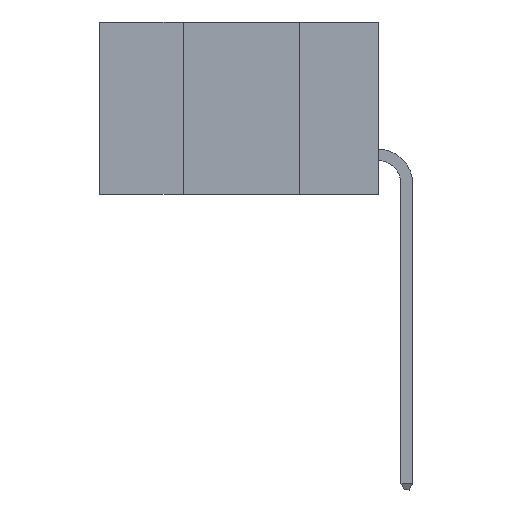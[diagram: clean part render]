
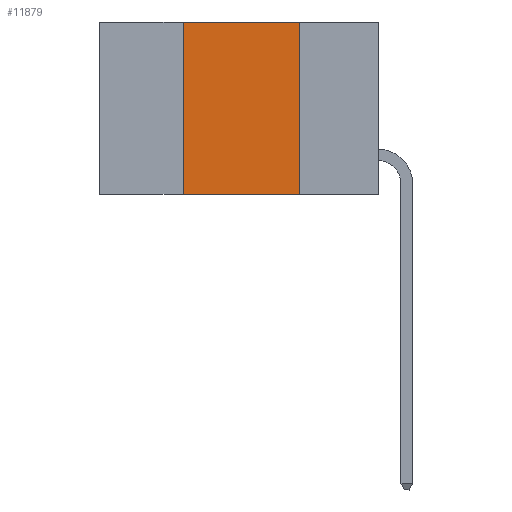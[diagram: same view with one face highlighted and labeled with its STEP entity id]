
A CAD part, left-side view. The second image highlights one B-rep face of the part: STEP entity #11879.
In plain terms, the highlighted planar face has unit normal (-1, 0, 0).
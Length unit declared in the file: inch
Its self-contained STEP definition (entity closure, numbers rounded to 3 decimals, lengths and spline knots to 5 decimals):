
#529 = VERTEX_POINT ( 'NONE', #8936 ) ;
#1614 = DIRECTION ( 'NONE',  ( 1., 0., 0. ) ) ;
#1861 = DIRECTION ( 'NONE',  ( 0., -1., 0. ) ) ;
#1899 = DIRECTION ( 'NONE',  ( 0., 0., -1. ) ) ;
#2452 = VECTOR ( 'NONE', #13883, 39.37008 ) ;
#2727 = EDGE_CURVE ( 'NONE', #3364, #13412, #4231, .T. ) ;
#3364 = VERTEX_POINT ( 'NONE', #25128 ) ;
#3997 = DIRECTION ( 'NONE',  ( 0., -1., 0. ) ) ;
#4231 = LINE ( 'NONE', #13384, #15746 ) ;
#4627 = CARTESIAN_POINT ( 'NONE',  ( 0., 0.17, 0. ) ) ;
#4944 = AXIS2_PLACEMENT_3D ( 'NONE', #15744, #1614, #1899 ) ;
#6671 = VECTOR ( 'NONE', #9051, 39.37008 ) ;
#7128 = VERTEX_POINT ( 'NONE', #12158 ) ;
#7624 = CARTESIAN_POINT ( 'NONE',  ( 0., 0.17, 0. ) ) ;
#8653 = FACE_OUTER_BOUND ( 'NONE', #9447, .T. ) ;
#8936 = CARTESIAN_POINT ( 'NONE',  ( 0., 0.42, -0.37 ) ) ;
#9051 = DIRECTION ( 'NONE',  ( 0., 0., 1. ) ) ;
#9306 = EDGE_CURVE ( 'NONE', #529, #3364, #20756, .T. ) ;
#9447 = EDGE_LOOP ( 'NONE', ( #17401, #18548, #25231, #12040 ) ) ;
#11284 = CARTESIAN_POINT ( 'NONE',  ( 0., 0.42, 0. ) ) ;
#11879 = ADVANCED_FACE ( 'NONE', ( #8653 ), #24726, .F. ) ;
#12040 = ORIENTED_EDGE ( 'NONE', *, *, #18620, .T. ) ;
#12158 = CARTESIAN_POINT ( 'NONE',  ( 0., 0.17, -0.37 ) ) ;
#13384 = CARTESIAN_POINT ( 'NONE',  ( 0., 0.6, 0. ) ) ;
#13412 = VERTEX_POINT ( 'NONE', #7624 ) ;
#13883 = DIRECTION ( 'NONE',  ( 0., 0., -1. ) ) ;
#15744 = CARTESIAN_POINT ( 'NONE',  ( 0., 0.6, 0. ) ) ;
#15746 = VECTOR ( 'NONE', #1861, 39.37008 ) ;
#17379 = CARTESIAN_POINT ( 'NONE',  ( 0., 0.6, -0.37 ) ) ;
#17401 = ORIENTED_EDGE ( 'NONE', *, *, #29142, .F. ) ;
#18066 = VECTOR ( 'NONE', #3997, 39.37008 ) ;
#18548 = ORIENTED_EDGE ( 'NONE', *, *, #2727, .F. ) ;
#18620 = EDGE_CURVE ( 'NONE', #529, #7128, #22829, .T. ) ;
#19451 = LINE ( 'NONE', #4627, #2452 ) ;
#20756 = LINE ( 'NONE', #11284, #6671 ) ;
#22829 = LINE ( 'NONE', #17379, #18066 ) ;
#24726 = PLANE ( 'NONE',  #4944 ) ;
#25128 = CARTESIAN_POINT ( 'NONE',  ( 0., 0.42, 0. ) ) ;
#25231 = ORIENTED_EDGE ( 'NONE', *, *, #9306, .F. ) ;
#29142 = EDGE_CURVE ( 'NONE', #13412, #7128, #19451, .T. ) ;
